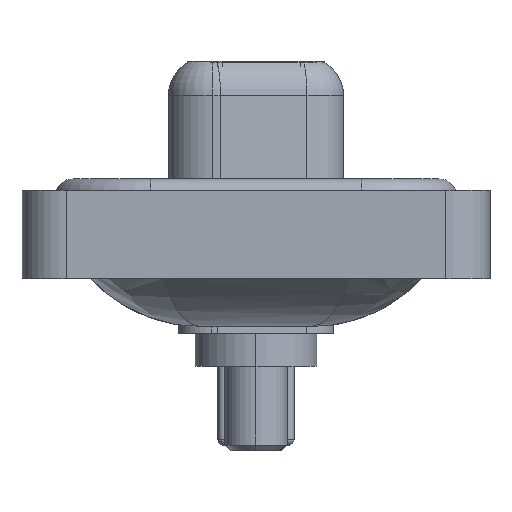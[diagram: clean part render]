
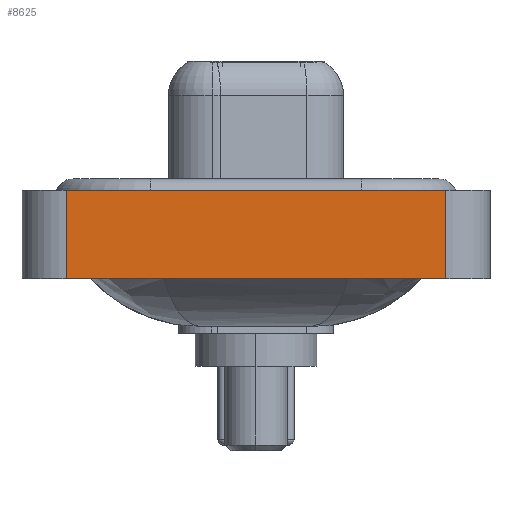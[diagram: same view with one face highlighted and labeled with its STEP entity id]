
A CAD part, left-side view. The second image highlights one B-rep face of the part: STEP entity #8625.
In plain terms, the highlighted planar face has unit normal (-1, 0, 0).
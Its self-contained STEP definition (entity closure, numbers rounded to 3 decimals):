
#170 = CARTESIAN_POINT ( 'NONE',  ( -7.35, -8.55, -3.6 ) ) ;
#171 = CARTESIAN_POINT ( 'NONE',  ( -7.35, 8.55, 0.4 ) ) ;
#355 = ORIENTED_EDGE ( 'NONE', *, *, #22415, .T. ) ;
#1285 = VERTEX_POINT ( 'NONE', #1388 ) ;
#1388 = CARTESIAN_POINT ( 'NONE',  ( -7.35, -8.55, 0.4 ) ) ;
#1572 = CARTESIAN_POINT ( 'NONE',  ( -7.35, 8.55, -3.6 ) ) ;
#2584 = EDGE_CURVE ( 'NONE', #7780, #1285, #13220, .T. ) ;
#3516 = DIRECTION ( 'NONE',  ( 0., 0., 1. ) ) ;
#3717 = DIRECTION ( 'NONE',  ( 0., -1., 0. ) ) ;
#4053 = EDGE_LOOP ( 'NONE', ( #355, #20449, #8633, #10826 ) ) ;
#4874 = DIRECTION ( 'NONE',  ( -1., 0., 0. ) ) ;
#5543 = VECTOR ( 'NONE', #12166, 1000. ) ;
#6503 = VECTOR ( 'NONE', #3717, 1000. ) ;
#6594 = LINE ( 'NONE', #1572, #12669 ) ;
#7780 = VERTEX_POINT ( 'NONE', #171 ) ;
#8071 = PLANE ( 'NONE',  #12683 ) ;
#8625 = ADVANCED_FACE ( 'NONE', ( #18641 ), #8071, .T. ) ;
#8633 = ORIENTED_EDGE ( 'NONE', *, *, #11858, .F. ) ;
#8990 = LINE ( 'NONE', #12506, #5543 ) ;
#9138 = CARTESIAN_POINT ( 'NONE',  ( -7.35, -8.55, -3.6 ) ) ;
#10538 = EDGE_CURVE ( 'NONE', #10781, #12340, #10640, .T. ) ;
#10640 = LINE ( 'NONE', #170, #6503 ) ;
#10781 = VERTEX_POINT ( 'NONE', #18137 ) ;
#10826 = ORIENTED_EDGE ( 'NONE', *, *, #10538, .T. ) ;
#11858 = EDGE_CURVE ( 'NONE', #10781, #7780, #6594, .T. ) ;
#12166 = DIRECTION ( 'NONE',  ( 0., 0., 1. ) ) ;
#12340 = VERTEX_POINT ( 'NONE', #9138 ) ;
#12506 = CARTESIAN_POINT ( 'NONE',  ( -7.35, -8.55, -3.6 ) ) ;
#12669 = VECTOR ( 'NONE', #3516, 1000. ) ;
#12683 = AXIS2_PLACEMENT_3D ( 'NONE', #22275, #4874, #20461 ) ;
#13220 = LINE ( 'NONE', #17087, #16956 ) ;
#16956 = VECTOR ( 'NONE', #20157, 1000. ) ;
#17087 = CARTESIAN_POINT ( 'NONE',  ( -7.35, -8.55, 0.4 ) ) ;
#18137 = CARTESIAN_POINT ( 'NONE',  ( -7.35, 8.55, -3.6 ) ) ;
#18641 = FACE_OUTER_BOUND ( 'NONE', #4053, .T. ) ;
#20157 = DIRECTION ( 'NONE',  ( 0., -1., 0. ) ) ;
#20449 = ORIENTED_EDGE ( 'NONE', *, *, #2584, .F. ) ;
#20461 = DIRECTION ( 'NONE',  ( 0., 0., 1. ) ) ;
#22275 = CARTESIAN_POINT ( 'NONE',  ( -7.35, -8.55, -3.6 ) ) ;
#22415 = EDGE_CURVE ( 'NONE', #12340, #1285, #8990, .T. ) ;
